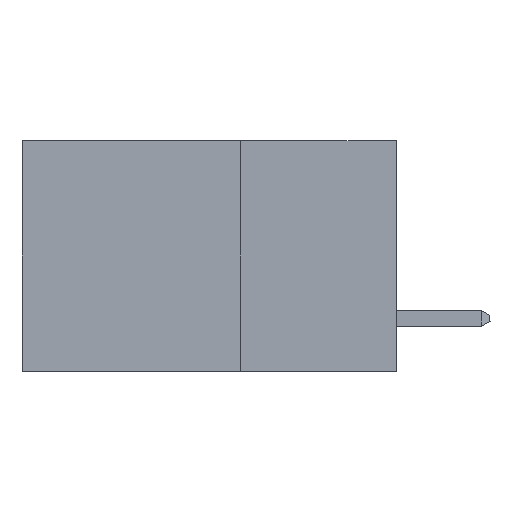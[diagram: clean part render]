
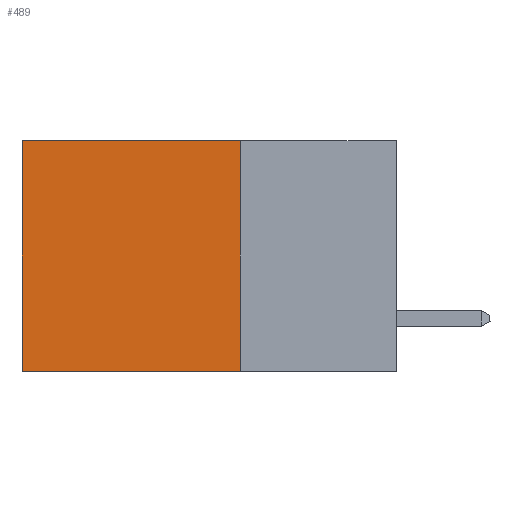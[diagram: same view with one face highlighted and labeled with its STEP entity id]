
A CAD part, left-side view. The second image highlights one B-rep face of the part: STEP entity #489.
In plain terms, the highlighted planar face has unit normal (-1, 0, 0).
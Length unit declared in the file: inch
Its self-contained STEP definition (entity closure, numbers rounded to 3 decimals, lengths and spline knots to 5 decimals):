
#366 = VERTEX_POINT ( 'NONE', #7874 ) ;
#385 = LINE ( 'NONE', #2981, #1014 ) ;
#434 = VERTEX_POINT ( 'NONE', #5805 ) ;
#489 = ADVANCED_FACE ( 'NONE', ( #7861 ), #4787, .F. ) ;
#749 = ORIENTED_EDGE ( 'NONE', *, *, #5565, .F. ) ;
#1014 = VECTOR ( 'NONE', #13449, 39.37008 ) ;
#1055 = CARTESIAN_POINT ( 'NONE',  ( 0.298, 0.6, 0. ) ) ;
#2207 = VECTOR ( 'NONE', #6858, 39.37008 ) ;
#2253 = ORIENTED_EDGE ( 'NONE', *, *, #15636, .F. ) ;
#2284 = DIRECTION ( 'NONE',  ( 0., 0., -1. ) ) ;
#2340 = DIRECTION ( 'NONE',  ( 1., 0., 0. ) ) ;
#2981 = CARTESIAN_POINT ( 'NONE',  ( 0.298, 0.25, 0. ) ) ;
#3181 = VECTOR ( 'NONE', #3289, 39.37008 ) ;
#3222 = VECTOR ( 'NONE', #3466, 39.37008 ) ;
#3289 = DIRECTION ( 'NONE',  ( 0., 1., 0. ) ) ;
#3378 = ORIENTED_EDGE ( 'NONE', *, *, #8008, .T. ) ;
#3466 = DIRECTION ( 'NONE',  ( 0., 0., -1. ) ) ;
#3803 = VERTEX_POINT ( 'NONE', #6329 ) ;
#4502 = CARTESIAN_POINT ( 'NONE',  ( 0.298, 0.25, -0.37 ) ) ;
#4787 = PLANE ( 'NONE',  #7990 ) ;
#5565 = EDGE_CURVE ( 'NONE', #434, #5761, #11284, .T. ) ;
#5761 = VERTEX_POINT ( 'NONE', #7814 ) ;
#5805 = CARTESIAN_POINT ( 'NONE',  ( 0.298, 0.25, 0. ) ) ;
#5881 = LINE ( 'NONE', #1055, #3222 ) ;
#6191 = EDGE_LOOP ( 'NONE', ( #9011, #2253, #749, #3378 ) ) ;
#6329 = CARTESIAN_POINT ( 'NONE',  ( 0.298, 0.6, 0. ) ) ;
#6858 = DIRECTION ( 'NONE',  ( 0., 0., -1. ) ) ;
#7814 = CARTESIAN_POINT ( 'NONE',  ( 0.298, 0.25, -0.37 ) ) ;
#7861 = FACE_OUTER_BOUND ( 'NONE', #6191, .T. ) ;
#7874 = CARTESIAN_POINT ( 'NONE',  ( 0.298, 0.6, -0.37 ) ) ;
#7990 = AXIS2_PLACEMENT_3D ( 'NONE', #8801, #2340, #2284 ) ;
#8008 = EDGE_CURVE ( 'NONE', #434, #3803, #385, .T. ) ;
#8801 = CARTESIAN_POINT ( 'NONE',  ( 0.298, 0.25, 0. ) ) ;
#9011 = ORIENTED_EDGE ( 'NONE', *, *, #9091, .T. ) ;
#9091 = EDGE_CURVE ( 'NONE', #3803, #366, #5881, .T. ) ;
#11284 = LINE ( 'NONE', #14851, #2207 ) ;
#12492 = LINE ( 'NONE', #4502, #3181 ) ;
#13449 = DIRECTION ( 'NONE',  ( 0., 1., 0. ) ) ;
#14851 = CARTESIAN_POINT ( 'NONE',  ( 0.298, 0.25, 0. ) ) ;
#15636 = EDGE_CURVE ( 'NONE', #5761, #366, #12492, .T. ) ;
